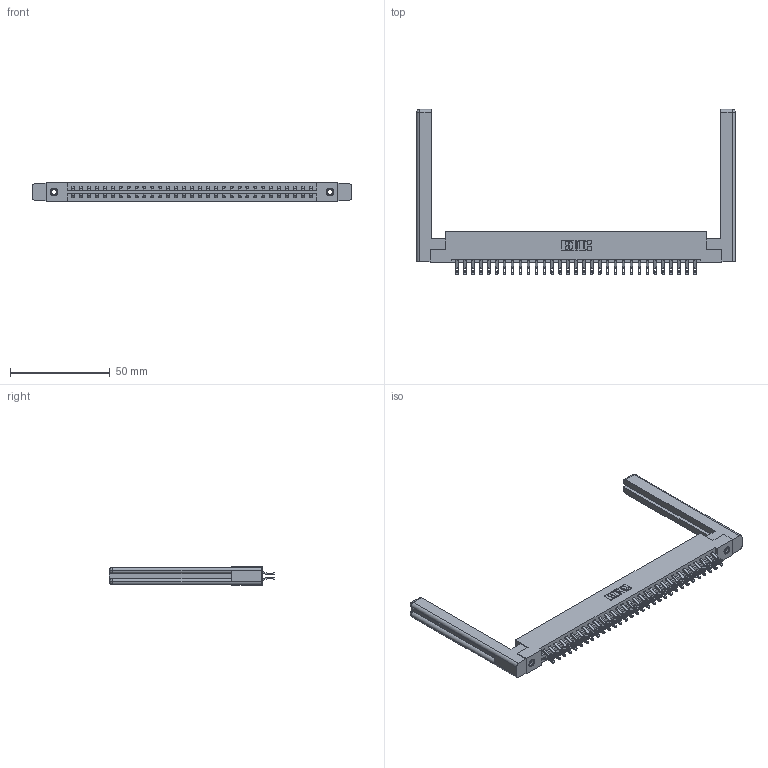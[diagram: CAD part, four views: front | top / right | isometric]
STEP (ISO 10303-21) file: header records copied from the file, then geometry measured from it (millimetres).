
FILE_DESCRIPTION (( 'STEP AP203' ), '1' );
FILE_NAME ('387-062-555-258.STEP', '2019-10-19T15:27:36', ( '' ), ( '' ), 'SwSTEP 2.0', 'SolidWorks 2016', '' );
FILE_SCHEMA (( 'CONFIG_CONTROL_DESIGN' ));
Length unit declared in the file: inch
Products named in the file (5): 345-250-001_345-250-001-102; 345-292-001_555 Tail; 387-062-555-258; 337 Part_Flush Mounting Lugs - 0.156 Dia-TI; 307-220-058
Assembly tree (67 placements, depth 2):
  387-062-555-258
    337 Part_Flush Mounting Lugs - 0.156 Dia-TI
    345-292-001_555 Tail  x62
    345-250-001_345-250-001-102  x2
    307-220-058  x2
Bounding box: 159.46 x 82.56 x 9.4 mm (x, y, z)
Volume: 23981 mm3; surface area: 24653.8 mm2
Topology: 67 solids, 67 shells, 3976 faces, 12383 edges, 8242 vertices
Faces by surface type: plane 2386, cylinder 1566, cone 12, torus 12
Entity records: 28418 total; most frequent: CARTESIAN_POINT 4839, ORIENTED_EDGE 4684, DIRECTION 4122, EDGE_CURVE 2342, VECTOR 2146, LINE 2146, VERTEX_POINT 1554, AXIS2_PLACEMENT_3D 988
